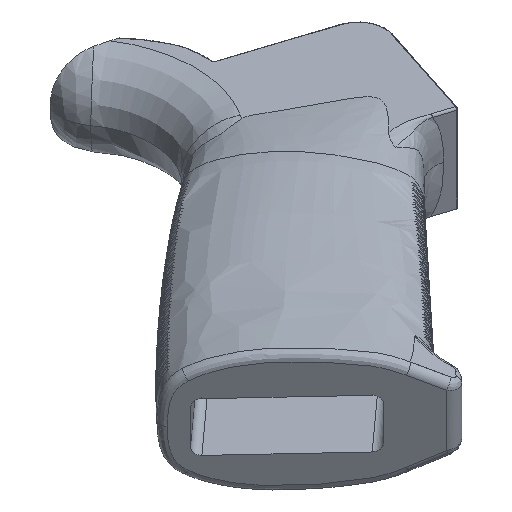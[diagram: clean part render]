
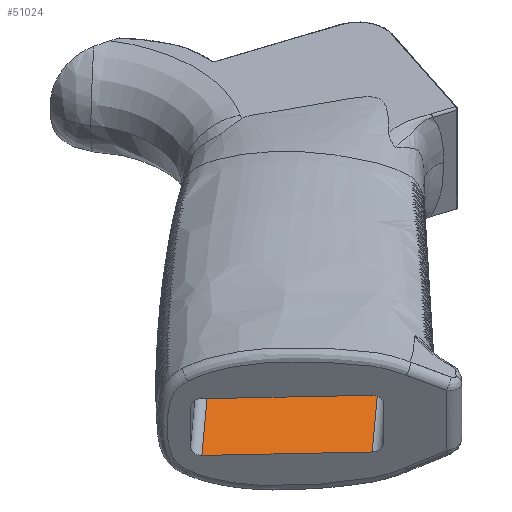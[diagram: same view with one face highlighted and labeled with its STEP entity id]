
A CAD part, isometric view. The second image highlights one B-rep face of the part: STEP entity #51024.
In plain terms, the highlighted planar face has unit normal (0, 0, 1).
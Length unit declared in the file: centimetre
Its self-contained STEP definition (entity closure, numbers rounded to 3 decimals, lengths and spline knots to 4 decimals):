
#3773 = CARTESIAN_POINT ( 'NONE',  ( -35.471, 27.7247, -0.5107 ) ) ;
#4367 = ORIENTED_EDGE ( 'NONE', *, *, #44813, .F. ) ;
#4429 = FACE_OUTER_BOUND ( 'NONE', #22264, .T. ) ;
#4819 = VERTEX_POINT ( 'NONE', #18761 ) ;
#5100 = VERTEX_POINT ( 'NONE', #38132 ) ;
#5700 = DIRECTION ( 'NONE',  ( -0.743, -0.669, 0. ) ) ;
#7148 = ORIENTED_EDGE ( 'NONE', *, *, #20005, .F. ) ;
#8488 = CARTESIAN_POINT ( 'NONE',  ( -31.4127, 31.3788, -0.5107 ) ) ;
#9347 = VECTOR ( 'NONE', #5700, 100. ) ;
#9422 = LINE ( 'NONE', #16418, #48213 ) ;
#9916 = LINE ( 'NONE', #13281, #21816 ) ;
#13281 = CARTESIAN_POINT ( 'NONE',  ( -28.492, 32.0741, -0.5107 ) ) ;
#14240 = VERTEX_POINT ( 'NONE', #18594 ) ;
#14304 = DIRECTION ( 'NONE',  ( 0.973, 0.232, 0. ) ) ;
#15572 = EDGE_CURVE ( 'NONE', #46786, #23411, #20636, .T. ) ;
#16418 = CARTESIAN_POINT ( 'NONE',  ( -27.7847, 31.2886, -0.5107 ) ) ;
#17361 = DIRECTION ( 'NONE',  ( 0., -1., 0. ) ) ;
#18548 = AXIS2_PLACEMENT_3D ( 'NONE', #25139, #36312, #17361 ) ;
#18594 = CARTESIAN_POINT ( 'NONE',  ( -27.7847, 31.2886, -0.5107 ) ) ;
#18761 = CARTESIAN_POINT ( 'NONE',  ( -33.2693, 25.6716, -0.5107 ) ) ;
#18813 = EDGE_CURVE ( 'NONE', #46786, #50758, #22585, .T. ) ;
#20005 = EDGE_CURVE ( 'NONE', #50758, #14240, #9916, .T. ) ;
#20108 = ORIENTED_EDGE ( 'NONE', *, *, #18813, .F. ) ;
#20636 = LINE ( 'NONE', #28918, #20894 ) ;
#20894 = VECTOR ( 'NONE', #33067, 100. ) ;
#21756 = CARTESIAN_POINT ( 'NONE',  ( -28.1183, 30.3095, -0.5107 ) ) ;
#21816 = VECTOR ( 'NONE', #29592, 100. ) ;
#22077 = CARTESIAN_POINT ( 'NONE',  ( -31.4127, 31.3788, -0.5107 ) ) ;
#22264 = EDGE_LOOP ( 'NONE', ( #48911, #41091, #4367, #23344, #7148, #20108 ) ) ;
#22585 = LINE ( 'NONE', #22077, #22638 ) ;
#22638 = VECTOR ( 'NONE', #14304, 100. ) ;
#23344 = ORIENTED_EDGE ( 'NONE', *, *, #40949, .F. ) ;
#23411 = VERTEX_POINT ( 'NONE', #3773 ) ;
#25139 = CARTESIAN_POINT ( 'NONE',  ( -34.7999, 24.0242, -0.5107 ) ) ;
#27650 = DIRECTION ( 'NONE',  ( -0.731, 0.682, 0. ) ) ;
#28918 = CARTESIAN_POINT ( 'NONE',  ( -36.9405, 26.4015, -0.5107 ) ) ;
#29592 = DIRECTION ( 'NONE',  ( 0.669, -0.743, 0. ) ) ;
#31791 = LINE ( 'NONE', #40085, #35867 ) ;
#32212 = DIRECTION ( 'NONE',  ( -0.322, -0.947, 0. ) ) ;
#32665 = PLANE ( 'NONE',  #18548 ) ;
#33067 = DIRECTION ( 'NONE',  ( -0.743, -0.669, 0. ) ) ;
#35867 = VECTOR ( 'NONE', #27650, 100. ) ;
#36312 = DIRECTION ( 'NONE',  ( 0., 0., -1. ) ) ;
#36830 = CARTESIAN_POINT ( 'NONE',  ( -28.492, 32.0741, -0.5107 ) ) ;
#38132 = CARTESIAN_POINT ( 'NONE',  ( -28.1183, 30.3095, -0.5107 ) ) ;
#40085 = CARTESIAN_POINT ( 'NONE',  ( -34.1743, 26.5155, -0.5107 ) ) ;
#40949 = EDGE_CURVE ( 'NONE', #14240, #5100, #9422, .T. ) ;
#41091 = ORIENTED_EDGE ( 'NONE', *, *, #45877, .F. ) ;
#44813 = EDGE_CURVE ( 'NONE', #5100, #4819, #45866, .T. ) ;
#45866 = LINE ( 'NONE', #21756, #9347 ) ;
#45877 = EDGE_CURVE ( 'NONE', #4819, #23411, #31791, .T. ) ;
#46786 = VERTEX_POINT ( 'NONE', #8488 ) ;
#48213 = VECTOR ( 'NONE', #32212, 100. ) ;
#48911 = ORIENTED_EDGE ( 'NONE', *, *, #15572, .T. ) ;
#50758 = VERTEX_POINT ( 'NONE', #36830 ) ;
#51024 = ADVANCED_FACE ( 'NONE', ( #4429 ), #32665, .F. ) ;
